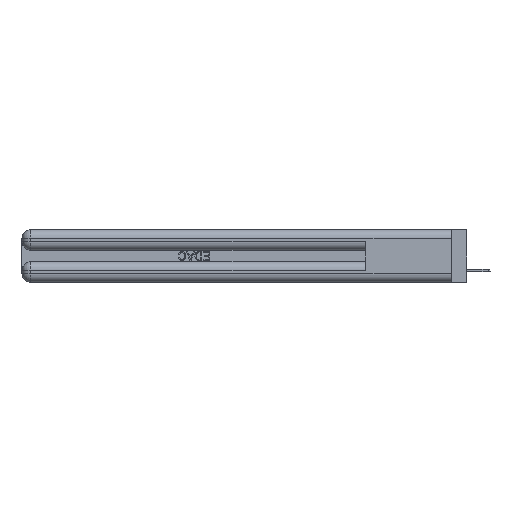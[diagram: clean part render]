
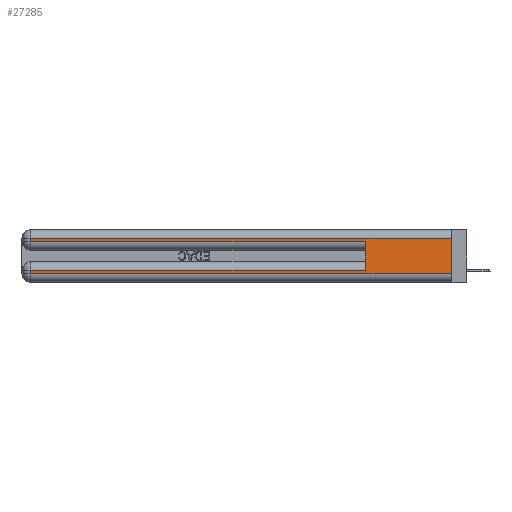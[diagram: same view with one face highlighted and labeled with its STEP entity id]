
A CAD part, left-side view. The second image highlights one B-rep face of the part: STEP entity #27285.
In plain terms, the highlighted planar face has unit normal (-1, 0, 0).
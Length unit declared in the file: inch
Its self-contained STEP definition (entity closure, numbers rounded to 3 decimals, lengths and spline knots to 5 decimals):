
#709 = LINE ( 'NONE', #39176, #34200 ) ;
#1181 = CARTESIAN_POINT ( 'NONE',  ( 0., 0., 0.06 ) ) ;
#3175 = CARTESIAN_POINT ( 'NONE',  ( 0., 0., 0.31 ) ) ;
#4455 = LINE ( 'NONE', #36882, #6273 ) ;
#5602 = VERTEX_POINT ( 'NONE', #26895 ) ;
#5768 = LINE ( 'NONE', #8659, #14757 ) ;
#6273 = VECTOR ( 'NONE', #44848, 39.37008 ) ;
#8459 = ORIENTED_EDGE ( 'NONE', *, *, #21588, .F. ) ;
#8659 = CARTESIAN_POINT ( 'NONE',  ( 0., 0.6, 0.145 ) ) ;
#9239 = VERTEX_POINT ( 'NONE', #3175 ) ;
#10737 = VERTEX_POINT ( 'NONE', #25830 ) ;
#11099 = CARTESIAN_POINT ( 'NONE',  ( 0., 2.94, 0.37 ) ) ;
#12550 = EDGE_CURVE ( 'NONE', #5602, #10737, #31889, .T. ) ;
#14757 = VECTOR ( 'NONE', #35487, 39.37008 ) ;
#15949 = VECTOR ( 'NONE', #32749, 39.37008 ) ;
#16520 = CARTESIAN_POINT ( 'NONE',  ( 0., 0., 0.37 ) ) ;
#16779 = EDGE_LOOP ( 'NONE', ( #18629, #37724, #47309, #41092, #8459, #32001, #28307, #20077 ) ) ;
#18629 = ORIENTED_EDGE ( 'NONE', *, *, #34798, .F. ) ;
#18685 = DIRECTION ( 'NONE',  ( 0., 1., 0. ) ) ;
#18691 = VERTEX_POINT ( 'NONE', #35401 ) ;
#20077 = ORIENTED_EDGE ( 'NONE', *, *, #36191, .T. ) ;
#20869 = DIRECTION ( 'NONE',  ( 0., 0., -1. ) ) ;
#21588 = EDGE_CURVE ( 'NONE', #5602, #38975, #5768, .T. ) ;
#23709 = LINE ( 'NONE', #36987, #15949 ) ;
#25195 = VERTEX_POINT ( 'NONE', #39775 ) ;
#25272 = AXIS2_PLACEMENT_3D ( 'NONE', #32332, #36375, #43526 ) ;
#25830 = CARTESIAN_POINT ( 'NONE',  ( 0., 2.94, 0.085 ) ) ;
#26053 = CARTESIAN_POINT ( 'NONE',  ( 0., 2.94, 0.31 ) ) ;
#26895 = CARTESIAN_POINT ( 'NONE',  ( 0., 0.6, 0.085 ) ) ;
#27285 = ADVANCED_FACE ( 'NONE', ( #29512 ), #43864, .F. ) ;
#27660 = DIRECTION ( 'NONE',  ( 0., 0., -1. ) ) ;
#27788 = EDGE_CURVE ( 'NONE', #30558, #25195, #709, .T. ) ;
#28307 = ORIENTED_EDGE ( 'NONE', *, *, #30925, .T. ) ;
#28311 = VECTOR ( 'NONE', #20869, 39.37008 ) ;
#29512 = FACE_OUTER_BOUND ( 'NONE', #16779, .T. ) ;
#30558 = VERTEX_POINT ( 'NONE', #26053 ) ;
#30925 = EDGE_CURVE ( 'NONE', #10737, #18691, #34842, .T. ) ;
#31660 = CARTESIAN_POINT ( 'NONE',  ( 0., 0., 0.085 ) ) ;
#31889 = LINE ( 'NONE', #31660, #32536 ) ;
#32001 = ORIENTED_EDGE ( 'NONE', *, *, #12550, .T. ) ;
#32032 = LINE ( 'NONE', #16520, #34990 ) ;
#32332 = CARTESIAN_POINT ( 'NONE',  ( 0., 0., 0.37 ) ) ;
#32536 = VECTOR ( 'NONE', #18685, 39.37008 ) ;
#32749 = DIRECTION ( 'NONE',  ( 0., 1., 0. ) ) ;
#32952 = VERTEX_POINT ( 'NONE', #43891 ) ;
#34200 = VECTOR ( 'NONE', #40358, 39.37008 ) ;
#34798 = EDGE_CURVE ( 'NONE', #9239, #32952, #32032, .T. ) ;
#34842 = LINE ( 'NONE', #11099, #28311 ) ;
#34990 = VECTOR ( 'NONE', #27660, 39.37008 ) ;
#35401 = CARTESIAN_POINT ( 'NONE',  ( 0., 2.94, 0.06 ) ) ;
#35487 = DIRECTION ( 'NONE',  ( 0., 0., 1. ) ) ;
#36191 = EDGE_CURVE ( 'NONE', #18691, #32952, #44759, .T. ) ;
#36375 = DIRECTION ( 'NONE',  ( 1., 0., 0. ) ) ;
#36882 = CARTESIAN_POINT ( 'NONE',  ( 0., 0., 0.285 ) ) ;
#36987 = CARTESIAN_POINT ( 'NONE',  ( 0., 0., 0.31 ) ) ;
#37724 = ORIENTED_EDGE ( 'NONE', *, *, #48754, .T. ) ;
#38975 = VERTEX_POINT ( 'NONE', #41193 ) ;
#39176 = CARTESIAN_POINT ( 'NONE',  ( 0., 2.94, 0.37 ) ) ;
#39775 = CARTESIAN_POINT ( 'NONE',  ( 0., 2.94, 0.285 ) ) ;
#40358 = DIRECTION ( 'NONE',  ( 0., 0., -1. ) ) ;
#41092 = ORIENTED_EDGE ( 'NONE', *, *, #43070, .T. ) ;
#41193 = CARTESIAN_POINT ( 'NONE',  ( 0., 0.6, 0.285 ) ) ;
#42329 = VECTOR ( 'NONE', #44093, 39.37008 ) ;
#43070 = EDGE_CURVE ( 'NONE', #25195, #38975, #4455, .T. ) ;
#43526 = DIRECTION ( 'NONE',  ( 0., 0., -1. ) ) ;
#43864 = PLANE ( 'NONE',  #25272 ) ;
#43891 = CARTESIAN_POINT ( 'NONE',  ( 0., 0., 0.06 ) ) ;
#44093 = DIRECTION ( 'NONE',  ( 0., -1., 0. ) ) ;
#44759 = LINE ( 'NONE', #1181, #42329 ) ;
#44848 = DIRECTION ( 'NONE',  ( 0., -1., 0. ) ) ;
#47309 = ORIENTED_EDGE ( 'NONE', *, *, #27788, .T. ) ;
#48754 = EDGE_CURVE ( 'NONE', #9239, #30558, #23709, .T. ) ;
